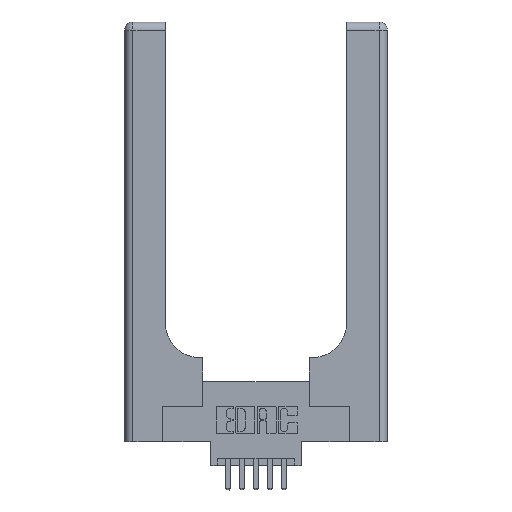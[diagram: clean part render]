
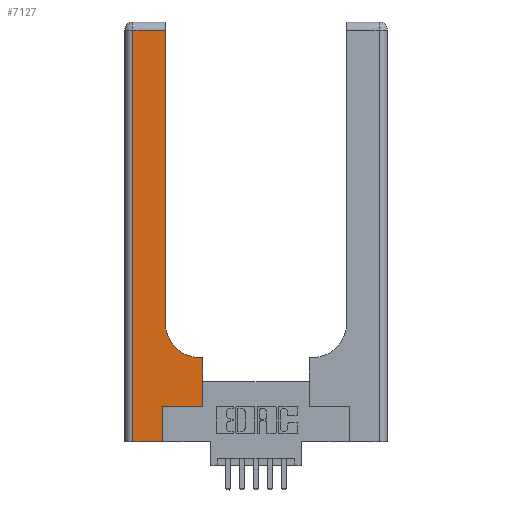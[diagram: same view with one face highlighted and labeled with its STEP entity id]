
A CAD part, top view. The second image highlights one B-rep face of the part: STEP entity #7127.
In plain terms, the highlighted planar face has unit normal (0, 0, 1).
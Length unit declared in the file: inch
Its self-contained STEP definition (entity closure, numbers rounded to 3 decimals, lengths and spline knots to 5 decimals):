
#34 = LINE ( 'NONE', #13669, #9588 ) ;
#73 = ORIENTED_EDGE ( 'NONE', *, *, #2083, .T. ) ;
#187 = DIRECTION ( 'NONE',  ( 0., 1., 0. ) ) ;
#244 = ORIENTED_EDGE ( 'NONE', *, *, #10111, .T. ) ;
#246 = DIRECTION ( 'NONE',  ( 1., 0., 0. ) ) ;
#248 = CARTESIAN_POINT ( 'NONE',  ( 0., 2.94, 0.37 ) ) ;
#381 = CARTESIAN_POINT ( 'NONE',  ( 0.5415, 0.6, 0.37 ) ) ;
#468 = VERTEX_POINT ( 'NONE', #10695 ) ;
#588 = VECTOR ( 'NONE', #187, 39.37008 ) ;
#607 = CARTESIAN_POINT ( 'NONE',  ( 0.5585, 0.25, 0.37 ) ) ;
#1062 = AXIS2_PLACEMENT_3D ( 'NONE', #4863, #11402, #246 ) ;
#1307 = CARTESIAN_POINT ( 'NONE',  ( 0.2915, 3., 0.37 ) ) ;
#1662 = DIRECTION ( 'NONE',  ( 0., 1., 0. ) ) ;
#1930 = VERTEX_POINT ( 'NONE', #381 ) ;
#1979 = DIRECTION ( 'NONE',  ( 1., 0., 0. ) ) ;
#2083 = EDGE_CURVE ( 'NONE', #9575, #13075, #11220, .T. ) ;
#2474 = CARTESIAN_POINT ( 'NONE',  ( 0.2915, 2.94, 0.37 ) ) ;
#2567 = VERTEX_POINT ( 'NONE', #3439 ) ;
#2621 = LINE ( 'NONE', #4318, #14071 ) ;
#3167 = ORIENTED_EDGE ( 'NONE', *, *, #3410, .T. ) ;
#3220 = CARTESIAN_POINT ( 'NONE',  ( 0.269, 0.25, 0.37 ) ) ;
#3410 = EDGE_CURVE ( 'NONE', #12867, #3946, #12555, .T. ) ;
#3436 = DIRECTION ( 'NONE',  ( 0., -1., 0. ) ) ;
#3439 = CARTESIAN_POINT ( 'NONE',  ( 0.5585, 0.25, 0.37 ) ) ;
#3946 = VERTEX_POINT ( 'NONE', #12658 ) ;
#4318 = CARTESIAN_POINT ( 'NONE',  ( 0.06, 3., 0.37 ) ) ;
#4489 = ORIENTED_EDGE ( 'NONE', *, *, #6201, .T. ) ;
#4863 = CARTESIAN_POINT ( 'NONE',  ( 0.5415, 0.85, 0.37 ) ) ;
#4893 = CARTESIAN_POINT ( 'NONE',  ( 0.269, 0., 0.37 ) ) ;
#5036 = LINE ( 'NONE', #607, #7312 ) ;
#5300 = VECTOR ( 'NONE', #10581, 39.37008 ) ;
#5803 = ORIENTED_EDGE ( 'NONE', *, *, #12241, .T. ) ;
#6096 = CARTESIAN_POINT ( 'NONE',  ( 0.2915, 0.85, 0.37 ) ) ;
#6201 = EDGE_CURVE ( 'NONE', #1930, #9467, #10017, .T. ) ;
#6496 = LINE ( 'NONE', #3220, #12897 ) ;
#7127 = ADVANCED_FACE ( 'NONE', ( #14306 ), #8129, .F. ) ;
#7312 = VECTOR ( 'NONE', #1662, 39.37008 ) ;
#7482 = CARTESIAN_POINT ( 'NONE',  ( 0.269, 0.25, 0.37 ) ) ;
#7502 = VECTOR ( 'NONE', #7815, 39.37008 ) ;
#7800 = EDGE_CURVE ( 'NONE', #8518, #2567, #6496, .T. ) ;
#7815 = DIRECTION ( 'NONE',  ( 0., 1., 0. ) ) ;
#7843 = LINE ( 'NONE', #9142, #7502 ) ;
#7984 = DIRECTION ( 'NONE',  ( 0., 0., -1. ) ) ;
#8129 = PLANE ( 'NONE',  #11604 ) ;
#8245 = ORIENTED_EDGE ( 'NONE', *, *, #12746, .T. ) ;
#8518 = VERTEX_POINT ( 'NONE', #7482 ) ;
#9008 = ORIENTED_EDGE ( 'NONE', *, *, #9201, .T. ) ;
#9061 = DIRECTION ( 'NONE',  ( -1., 0., 0. ) ) ;
#9142 = CARTESIAN_POINT ( 'NONE',  ( 0.269, 0., 0.37 ) ) ;
#9201 = EDGE_CURVE ( 'NONE', #468, #1930, #34, .T. ) ;
#9467 = VERTEX_POINT ( 'NONE', #6096 ) ;
#9575 = VERTEX_POINT ( 'NONE', #13586 ) ;
#9588 = VECTOR ( 'NONE', #13525, 39.37008 ) ;
#9800 = EDGE_CURVE ( 'NONE', #2567, #468, #5036, .T. ) ;
#9978 = ORIENTED_EDGE ( 'NONE', *, *, #7800, .T. ) ;
#10017 = CIRCLE ( 'NONE', #1062, 0.25 ) ;
#10111 = EDGE_CURVE ( 'NONE', #13075, #8518, #7843, .T. ) ;
#10314 = CARTESIAN_POINT ( 'NONE',  ( 0., 3., 0.37 ) ) ;
#10581 = DIRECTION ( 'NONE',  ( 1., 0., 0. ) ) ;
#10695 = CARTESIAN_POINT ( 'NONE',  ( 0.5585, 0.6, 0.37 ) ) ;
#11220 = LINE ( 'NONE', #12913, #5300 ) ;
#11402 = DIRECTION ( 'NONE',  ( 0., 0., -1. ) ) ;
#11604 = AXIS2_PLACEMENT_3D ( 'NONE', #10314, #7984, #9061 ) ;
#12241 = EDGE_CURVE ( 'NONE', #9467, #12867, #13413, .T. ) ;
#12344 = EDGE_LOOP ( 'NONE', ( #5803, #3167, #8245, #73, #244, #9978, #12922, #9008, #4489 ) ) ;
#12555 = LINE ( 'NONE', #248, #14284 ) ;
#12658 = CARTESIAN_POINT ( 'NONE',  ( 0.06, 2.94, 0.37 ) ) ;
#12746 = EDGE_CURVE ( 'NONE', #3946, #9575, #2621, .T. ) ;
#12867 = VERTEX_POINT ( 'NONE', #2474 ) ;
#12897 = VECTOR ( 'NONE', #1979, 39.37008 ) ;
#12913 = CARTESIAN_POINT ( 'NONE',  ( 0., 0., 0.37 ) ) ;
#12922 = ORIENTED_EDGE ( 'NONE', *, *, #9800, .T. ) ;
#13075 = VERTEX_POINT ( 'NONE', #4893 ) ;
#13413 = LINE ( 'NONE', #1307, #588 ) ;
#13525 = DIRECTION ( 'NONE',  ( -1., 0., 0. ) ) ;
#13586 = CARTESIAN_POINT ( 'NONE',  ( 0.06, 0., 0.37 ) ) ;
#13669 = CARTESIAN_POINT ( 'NONE',  ( 0.2915, 0.6, 0.37 ) ) ;
#13688 = DIRECTION ( 'NONE',  ( -1., 0., 0. ) ) ;
#14071 = VECTOR ( 'NONE', #3436, 39.37008 ) ;
#14284 = VECTOR ( 'NONE', #13688, 39.37008 ) ;
#14306 = FACE_OUTER_BOUND ( 'NONE', #12344, .T. ) ;
